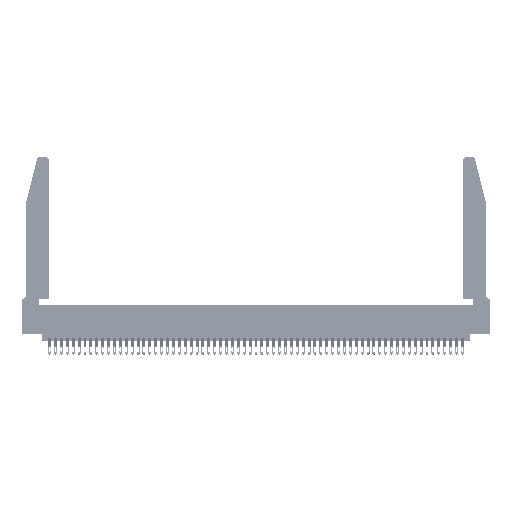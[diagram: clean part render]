
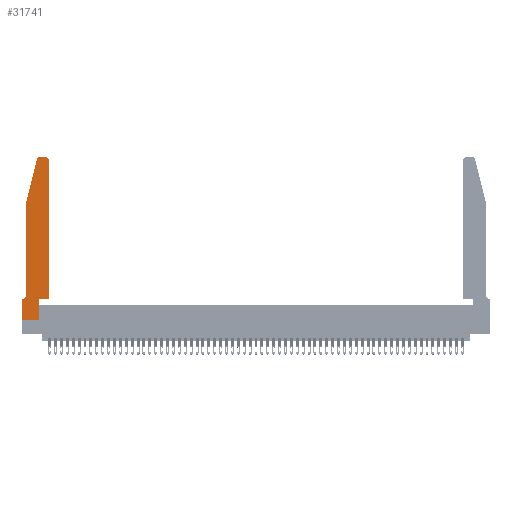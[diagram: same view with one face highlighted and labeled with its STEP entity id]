
A CAD part, top view. The second image highlights one B-rep face of the part: STEP entity #31741.
In plain terms, the highlighted planar face has unit normal (0, 0, 1).
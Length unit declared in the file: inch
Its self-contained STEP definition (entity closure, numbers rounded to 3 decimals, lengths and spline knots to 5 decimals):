
#69 = VERTEX_POINT ( 'NONE', #55637 ) ;
#1234 = CIRCLE ( 'NONE', #49501, 0.03 ) ;
#1804 = DIRECTION ( 'NONE',  ( 0., -1., 0. ) ) ;
#2611 = ORIENTED_EDGE ( 'NONE', *, *, #54640, .T. ) ;
#2844 = VERTEX_POINT ( 'NONE', #41818 ) ;
#4131 = DIRECTION ( 'NONE',  ( 1., 0., 0. ) ) ;
#4137 = CARTESIAN_POINT ( 'NONE',  ( 0., 0., 0.37 ) ) ;
#4617 = EDGE_CURVE ( 'NONE', #52672, #13261, #8168, .T. ) ;
#4797 = ORIENTED_EDGE ( 'NONE', *, *, #34259, .T. ) ;
#5222 = CARTESIAN_POINT ( 'NONE',  ( 0.0055, 0.42, 0.37 ) ) ;
#6072 = VERTEX_POINT ( 'NONE', #32821 ) ;
#6229 = CARTESIAN_POINT ( 'NONE',  ( 0.284, 2.75, 0.37 ) ) ;
#6516 = DIRECTION ( 'NONE',  ( -1., 0., 0. ) ) ;
#7794 = ORIENTED_EDGE ( 'NONE', *, *, #29237, .T. ) ;
#8049 = DIRECTION ( 'NONE',  ( 1., 0., 0. ) ) ;
#8168 = LINE ( 'NONE', #9972, #52279 ) ;
#8177 = ORIENTED_EDGE ( 'NONE', *, *, #14891, .T. ) ;
#8185 = VECTOR ( 'NONE', #25496, 39.37008 ) ;
#8247 = AXIS2_PLACEMENT_3D ( 'NONE', #5222, #36129, #9674 ) ;
#8457 = DIRECTION ( 'NONE',  ( 0., 1., 0. ) ) ;
#8602 = DIRECTION ( 'NONE',  ( 1., 0., 0. ) ) ;
#9549 = LINE ( 'NONE', #51798, #8185 ) ;
#9674 = DIRECTION ( 'NONE',  ( -1., 0., 0. ) ) ;
#9972 = CARTESIAN_POINT ( 'NONE',  ( 0.4505, 0.35, 0.37 ) ) ;
#11785 = ORIENTED_EDGE ( 'NONE', *, *, #14734, .T. ) ;
#12890 = CARTESIAN_POINT ( 'NONE',  ( 0.4505, 0.35, 0.37 ) ) ;
#13261 = VERTEX_POINT ( 'NONE', #15361 ) ;
#14515 = EDGE_CURVE ( 'NONE', #69, #41803, #29652, .T. ) ;
#14734 = EDGE_CURVE ( 'NONE', #29961, #55681, #9549, .T. ) ;
#14891 = EDGE_CURVE ( 'NONE', #46132, #69, #1234, .T. ) ;
#14973 = CARTESIAN_POINT ( 'NONE',  ( 0.0055, 0.35, 0.37 ) ) ;
#15361 = CARTESIAN_POINT ( 'NONE',  ( 0.4505, 0.35, 0.37 ) ) ;
#16529 = EDGE_LOOP ( 'NONE', ( #53600, #48037, #11785, #45454, #7794, #20206, #51273, #2611, #4797, #28876, #38597, #8177 ) ) ;
#16706 = CARTESIAN_POINT ( 'NONE',  ( 0., 0., 0.37 ) ) ;
#18636 = CARTESIAN_POINT ( 'NONE',  ( 0.4505, 2.72, 0.37 ) ) ;
#19118 = CIRCLE ( 'NONE', #32592, 0.03 ) ;
#20206 = ORIENTED_EDGE ( 'NONE', *, *, #44430, .T. ) ;
#20651 = VECTOR ( 'NONE', #6516, 39.37008 ) ;
#21011 = CARTESIAN_POINT ( 'NONE',  ( 0.2865, 0., 0.37 ) ) ;
#21257 = DIRECTION ( 'NONE',  ( 0., -1., 0. ) ) ;
#22207 = CARTESIAN_POINT ( 'NONE',  ( 0.0755, 0.35, 0.37 ) ) ;
#24142 = CARTESIAN_POINT ( 'NONE',  ( 0.0755, 2., 0.37 ) ) ;
#24336 = LINE ( 'NONE', #56271, #46361 ) ;
#24539 = DIRECTION ( 'NONE',  ( 0., 1., 0. ) ) ;
#24864 = DIRECTION ( 'NONE',  ( 0., 0., 1. ) ) ;
#25496 = DIRECTION ( 'NONE',  ( -0.239, -0.971, 0. ) ) ;
#25666 = CARTESIAN_POINT ( 'NONE',  ( 0., 0.35, 0.37 ) ) ;
#25802 = LINE ( 'NONE', #41343, #27171 ) ;
#27171 = VECTOR ( 'NONE', #1804, 39.37008 ) ;
#28729 = LINE ( 'NONE', #46646, #39030 ) ;
#28876 = ORIENTED_EDGE ( 'NONE', *, *, #4617, .T. ) ;
#29237 = EDGE_CURVE ( 'NONE', #2844, #46232, #55670, .T. ) ;
#29652 = LINE ( 'NONE', #32992, #20651 ) ;
#29961 = VERTEX_POINT ( 'NONE', #30822 ) ;
#30077 = PLANE ( 'NONE',  #34190 ) ;
#30319 = FACE_OUTER_BOUND ( 'NONE', #16529, .T. ) ;
#30629 = DIRECTION ( 'NONE',  ( 0., 0., 1. ) ) ;
#30822 = CARTESIAN_POINT ( 'NONE',  ( 0.25487, 2.72718, 0.37 ) ) ;
#31540 = VECTOR ( 'NONE', #8602, 39.37008 ) ;
#31741 = ADVANCED_FACE ( 'NONE', ( #30319 ), #30077, .T. ) ;
#32592 = AXIS2_PLACEMENT_3D ( 'NONE', #51187, #24864, #55606 ) ;
#32821 = CARTESIAN_POINT ( 'NONE',  ( 0., 0.35, 0.37 ) ) ;
#32992 = CARTESIAN_POINT ( 'NONE',  ( 0.2605, 2.75, 0.37 ) ) ;
#33412 = LINE ( 'NONE', #22207, #43712 ) ;
#34190 = AXIS2_PLACEMENT_3D ( 'NONE', #25666, #34495, #8049 ) ;
#34259 = EDGE_CURVE ( 'NONE', #50196, #52672, #28729, .T. ) ;
#34495 = DIRECTION ( 'NONE',  ( 0., 0., 1. ) ) ;
#36129 = DIRECTION ( 'NONE',  ( 0., 0., -1. ) ) ;
#38597 = ORIENTED_EDGE ( 'NONE', *, *, #50313, .T. ) ;
#39030 = VECTOR ( 'NONE', #24539, 39.37008 ) ;
#40900 = VECTOR ( 'NONE', #8457, 39.37008 ) ;
#41343 = CARTESIAN_POINT ( 'NONE',  ( 0.0755, 2., 0.37 ) ) ;
#41802 = EDGE_CURVE ( 'NONE', #55681, #2844, #25802, .T. ) ;
#41803 = VERTEX_POINT ( 'NONE', #6229 ) ;
#41818 = CARTESIAN_POINT ( 'NONE',  ( 0.0755, 0.42, 0.37 ) ) ;
#42285 = EDGE_CURVE ( 'NONE', #6072, #54550, #24336, .T. ) ;
#43712 = VECTOR ( 'NONE', #52992, 39.37008 ) ;
#44430 = EDGE_CURVE ( 'NONE', #46232, #6072, #33412, .T. ) ;
#45454 = ORIENTED_EDGE ( 'NONE', *, *, #41802, .T. ) ;
#46132 = VERTEX_POINT ( 'NONE', #18636 ) ;
#46232 = VERTEX_POINT ( 'NONE', #14973 ) ;
#46361 = VECTOR ( 'NONE', #21257, 39.37008 ) ;
#46646 = CARTESIAN_POINT ( 'NONE',  ( 0.2865, 0.35, 0.37 ) ) ;
#48037 = ORIENTED_EDGE ( 'NONE', *, *, #54450, .T. ) ;
#49501 = AXIS2_PLACEMENT_3D ( 'NONE', #56917, #30629, #4131 ) ;
#49682 = DIRECTION ( 'NONE',  ( 1., 0., 0. ) ) ;
#50196 = VERTEX_POINT ( 'NONE', #21011 ) ;
#50313 = EDGE_CURVE ( 'NONE', #13261, #46132, #53944, .T. ) ;
#51187 = CARTESIAN_POINT ( 'NONE',  ( 0.284, 2.72, 0.37 ) ) ;
#51273 = ORIENTED_EDGE ( 'NONE', *, *, #42285, .T. ) ;
#51736 = CARTESIAN_POINT ( 'NONE',  ( 0.2865, 0.35, 0.37 ) ) ;
#51798 = CARTESIAN_POINT ( 'NONE',  ( 0.0755, 2., 0.37 ) ) ;
#52279 = VECTOR ( 'NONE', #49682, 39.37008 ) ;
#52672 = VERTEX_POINT ( 'NONE', #51736 ) ;
#52992 = DIRECTION ( 'NONE',  ( -1., 0., 0. ) ) ;
#53600 = ORIENTED_EDGE ( 'NONE', *, *, #14515, .T. ) ;
#53944 = LINE ( 'NONE', #12890, #40900 ) ;
#54450 = EDGE_CURVE ( 'NONE', #41803, #29961, #19118, .T. ) ;
#54550 = VERTEX_POINT ( 'NONE', #16706 ) ;
#54640 = EDGE_CURVE ( 'NONE', #54550, #50196, #54932, .T. ) ;
#54932 = LINE ( 'NONE', #4137, #31540 ) ;
#55606 = DIRECTION ( 'NONE',  ( 1., 0., 0. ) ) ;
#55637 = CARTESIAN_POINT ( 'NONE',  ( 0.4205, 2.75, 0.37 ) ) ;
#55670 = CIRCLE ( 'NONE', #8247, 0.07 ) ;
#55681 = VERTEX_POINT ( 'NONE', #24142 ) ;
#56271 = CARTESIAN_POINT ( 'NONE',  ( 0., 0., 0.37 ) ) ;
#56917 = CARTESIAN_POINT ( 'NONE',  ( 0.4205, 2.72, 0.37 ) ) ;
